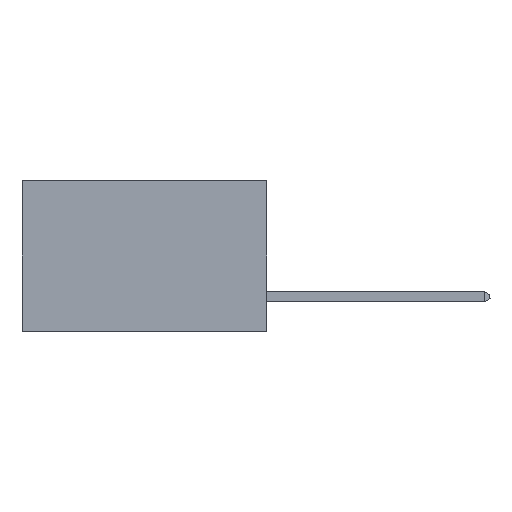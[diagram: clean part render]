
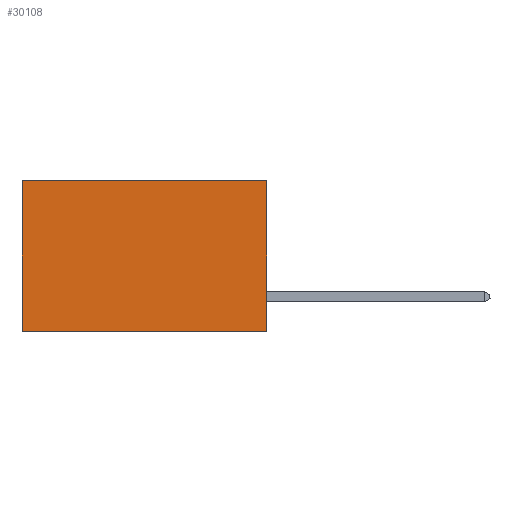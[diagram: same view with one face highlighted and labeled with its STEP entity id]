
A CAD part, left-side view. The second image highlights one B-rep face of the part: STEP entity #30108.
In plain terms, the highlighted planar face has unit normal (-1, 0, 0).
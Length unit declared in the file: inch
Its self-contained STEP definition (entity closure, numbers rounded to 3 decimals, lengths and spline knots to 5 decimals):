
#1842 = LINE ( 'NONE', #29451, #24936 ) ;
#2446 = EDGE_CURVE ( 'NONE', #39376, #36177, #4638, .T. ) ;
#3148 = VECTOR ( 'NONE', #25367, 39.37008 ) ;
#4209 = CARTESIAN_POINT ( 'NONE',  ( 0.2875, 0.6, 0. ) ) ;
#4638 = LINE ( 'NONE', #14949, #3148 ) ;
#6415 = ORIENTED_EDGE ( 'NONE', *, *, #32926, .T. ) ;
#6768 = EDGE_CURVE ( 'NONE', #36177, #23290, #1842, .T. ) ;
#7133 = FACE_OUTER_BOUND ( 'NONE', #24778, .T. ) ;
#7949 = CARTESIAN_POINT ( 'NONE',  ( 0.2875, 0.6, 0. ) ) ;
#8008 = CARTESIAN_POINT ( 'NONE',  ( 0.2875, 0., 0. ) ) ;
#8588 = DIRECTION ( 'NONE',  ( 0., 1., 0. ) ) ;
#9494 = ORIENTED_EDGE ( 'NONE', *, *, #34505, .T. ) ;
#14949 = CARTESIAN_POINT ( 'NONE',  ( 0.2875, 0., 0. ) ) ;
#16391 = DIRECTION ( 'NONE',  ( 0., 1., 0. ) ) ;
#16695 = PLANE ( 'NONE',  #36274 ) ;
#17372 = DIRECTION ( 'NONE',  ( 0., 0., -1. ) ) ;
#18396 = VERTEX_POINT ( 'NONE', #4209 ) ;
#19597 = VECTOR ( 'NONE', #8588, 39.37008 ) ;
#21973 = CARTESIAN_POINT ( 'NONE',  ( 0.2875, 0.6, -0.37 ) ) ;
#23011 = CARTESIAN_POINT ( 'NONE',  ( 0.2875, 0., -0.37 ) ) ;
#23290 = VERTEX_POINT ( 'NONE', #21973 ) ;
#23331 = ORIENTED_EDGE ( 'NONE', *, *, #6768, .F. ) ;
#23544 = LINE ( 'NONE', #7949, #33330 ) ;
#24778 = EDGE_LOOP ( 'NONE', ( #9494, #23331, #32854, #6415 ) ) ;
#24936 = VECTOR ( 'NONE', #16391, 39.37008 ) ;
#25367 = DIRECTION ( 'NONE',  ( 0., 0., -1. ) ) ;
#26308 = CARTESIAN_POINT ( 'NONE',  ( 0.2875, 0., 0. ) ) ;
#29451 = CARTESIAN_POINT ( 'NONE',  ( 0.2875, 0., -0.37 ) ) ;
#30018 = DIRECTION ( 'NONE',  ( 1., 0., 0. ) ) ;
#30108 = ADVANCED_FACE ( 'NONE', ( #7133 ), #16695, .F. ) ;
#30288 = CARTESIAN_POINT ( 'NONE',  ( 0.2875, 0., 0. ) ) ;
#32854 = ORIENTED_EDGE ( 'NONE', *, *, #2446, .F. ) ;
#32926 = EDGE_CURVE ( 'NONE', #39376, #18396, #39084, .T. ) ;
#33330 = VECTOR ( 'NONE', #34202, 39.37008 ) ;
#34202 = DIRECTION ( 'NONE',  ( 0., 0., -1. ) ) ;
#34505 = EDGE_CURVE ( 'NONE', #18396, #23290, #23544, .T. ) ;
#36177 = VERTEX_POINT ( 'NONE', #23011 ) ;
#36274 = AXIS2_PLACEMENT_3D ( 'NONE', #30288, #30018, #17372 ) ;
#39084 = LINE ( 'NONE', #8008, #19597 ) ;
#39376 = VERTEX_POINT ( 'NONE', #26308 ) ;
